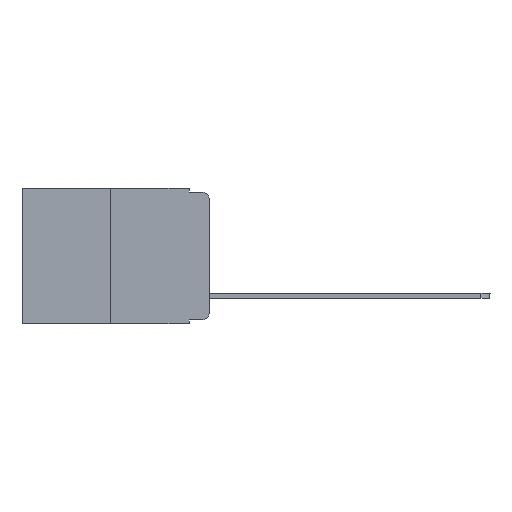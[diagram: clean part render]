
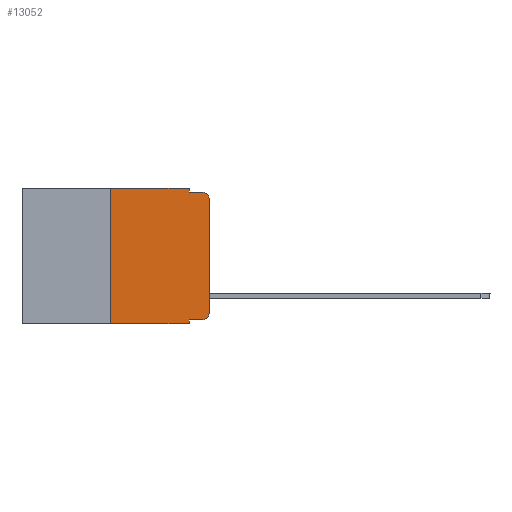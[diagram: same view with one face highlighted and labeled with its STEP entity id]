
A CAD part, left-side view. The second image highlights one B-rep face of the part: STEP entity #13052.
In plain terms, the highlighted planar face has unit normal (-1, 0, 0).
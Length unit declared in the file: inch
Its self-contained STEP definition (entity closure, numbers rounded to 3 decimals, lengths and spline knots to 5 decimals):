
#241 = DIRECTION ( 'NONE',  ( 0., 0., -1. ) ) ;
#373 = AXIS2_PLACEMENT_3D ( 'NONE', #2041, #6802, #15355 ) ;
#389 = VERTEX_POINT ( 'NONE', #5889 ) ;
#414 = EDGE_CURVE ( 'NONE', #12207, #12859, #4036, .T. ) ;
#885 = EDGE_CURVE ( 'NONE', #7667, #11808, #3461, .T. ) ;
#912 = PLANE ( 'NONE',  #373 ) ;
#1084 = DIRECTION ( 'NONE',  ( 0., 0., -1. ) ) ;
#1379 = DIRECTION ( 'NONE',  ( 0., -1., 0. ) ) ;
#1513 = CIRCLE ( 'NONE', #11182, 0.02 ) ;
#1989 = LINE ( 'NONE', #3856, #6149 ) ;
#2041 = CARTESIAN_POINT ( 'NONE',  ( 0., 0.473, 0. ) ) ;
#2101 = VERTEX_POINT ( 'NONE', #2649 ) ;
#2349 = CARTESIAN_POINT ( 'NONE',  ( 0., 0.473, 0. ) ) ;
#2479 = LINE ( 'NONE', #2349, #9505 ) ;
#2649 = CARTESIAN_POINT ( 'NONE',  ( 0., 0.02, -0.01 ) ) ;
#2656 = DIRECTION ( 'NONE',  ( 0., 0., 1. ) ) ;
#2687 = ORIENTED_EDGE ( 'NONE', *, *, #15153, .F. ) ;
#2711 = CARTESIAN_POINT ( 'NONE',  ( 0., 0.051, -0.333 ) ) ;
#3238 = CARTESIAN_POINT ( 'NONE',  ( 0., 0., -0.313 ) ) ;
#3398 = ORIENTED_EDGE ( 'NONE', *, *, #10942, .F. ) ;
#3461 = LINE ( 'NONE', #14426, #13952 ) ;
#3541 = VERTEX_POINT ( 'NONE', #10779 ) ;
#3684 = CARTESIAN_POINT ( 'NONE',  ( 0., 0.051, -0.343 ) ) ;
#3731 = EDGE_CURVE ( 'NONE', #13815, #2101, #1989, .T. ) ;
#3856 = CARTESIAN_POINT ( 'NONE',  ( 0., 0.051, -0.01 ) ) ;
#3975 = CARTESIAN_POINT ( 'NONE',  ( 0., 0.051, 0. ) ) ;
#4036 = LINE ( 'NONE', #10794, #9771 ) ;
#4743 = DIRECTION ( 'NONE',  ( -1., 0., 0. ) ) ;
#5081 = DIRECTION ( 'NONE',  ( 0., -1., 0. ) ) ;
#5144 = CARTESIAN_POINT ( 'NONE',  ( 0., 0.25, 0. ) ) ;
#5192 = ORIENTED_EDGE ( 'NONE', *, *, #9094, .F. ) ;
#5244 = VECTOR ( 'NONE', #2656, 39.37008 ) ;
#5296 = CARTESIAN_POINT ( 'NONE',  ( 0., 0.25, 0. ) ) ;
#5562 = LINE ( 'NONE', #3975, #13790 ) ;
#5621 = ORIENTED_EDGE ( 'NONE', *, *, #6258, .F. ) ;
#5871 = DIRECTION ( 'NONE',  ( 0., 0., -1. ) ) ;
#5889 = CARTESIAN_POINT ( 'NONE',  ( 0., 0.051, 0. ) ) ;
#5931 = DIRECTION ( 'NONE',  ( 0., 0., 1. ) ) ;
#6050 = DIRECTION ( 'NONE',  ( 0., -1., 0. ) ) ;
#6149 = VECTOR ( 'NONE', #5081, 39.37008 ) ;
#6258 = EDGE_CURVE ( 'NONE', #10572, #389, #2479, .T. ) ;
#6802 = DIRECTION ( 'NONE',  ( 1., 0., 0. ) ) ;
#6952 = EDGE_CURVE ( 'NONE', #11808, #2101, #8208, .T. ) ;
#7054 = ORIENTED_EDGE ( 'NONE', *, *, #11529, .T. ) ;
#7199 = VECTOR ( 'NONE', #1379, 39.37008 ) ;
#7667 = VERTEX_POINT ( 'NONE', #3238 ) ;
#7841 = ORIENTED_EDGE ( 'NONE', *, *, #3731, .F. ) ;
#8208 = CIRCLE ( 'NONE', #9423, 0.02 ) ;
#8435 = DIRECTION ( 'NONE',  ( 0., 0., -1. ) ) ;
#8578 = ORIENTED_EDGE ( 'NONE', *, *, #6952, .T. ) ;
#8870 = LINE ( 'NONE', #5144, #5244 ) ;
#9094 = EDGE_CURVE ( 'NONE', #389, #13815, #5562, .T. ) ;
#9423 = AXIS2_PLACEMENT_3D ( 'NONE', #10717, #13188, #5871 ) ;
#9505 = VECTOR ( 'NONE', #10631, 39.37008 ) ;
#9705 = LINE ( 'NONE', #14476, #15844 ) ;
#9771 = VECTOR ( 'NONE', #6050, 39.37008 ) ;
#10019 = CARTESIAN_POINT ( 'NONE',  ( 0., 0.473, -0.343 ) ) ;
#10572 = VERTEX_POINT ( 'NONE', #5296 ) ;
#10631 = DIRECTION ( 'NONE',  ( 0., -1., 0. ) ) ;
#10717 = CARTESIAN_POINT ( 'NONE',  ( 0., 0.02, -0.03 ) ) ;
#10779 = CARTESIAN_POINT ( 'NONE',  ( 0., 0.25, -0.343 ) ) ;
#10794 = CARTESIAN_POINT ( 'NONE',  ( 0., 0.051, -0.333 ) ) ;
#10815 = CARTESIAN_POINT ( 'NONE',  ( 0., 0.02, -0.313 ) ) ;
#10942 = EDGE_CURVE ( 'NONE', #12207, #11616, #9705, .T. ) ;
#11182 = AXIS2_PLACEMENT_3D ( 'NONE', #10815, #4743, #1084 ) ;
#11529 = EDGE_CURVE ( 'NONE', #12859, #7667, #1513, .T. ) ;
#11616 = VERTEX_POINT ( 'NONE', #3684 ) ;
#11798 = ORIENTED_EDGE ( 'NONE', *, *, #414, .T. ) ;
#11808 = VERTEX_POINT ( 'NONE', #13762 ) ;
#12207 = VERTEX_POINT ( 'NONE', #2711 ) ;
#12859 = VERTEX_POINT ( 'NONE', #13763 ) ;
#13052 = ADVANCED_FACE ( 'NONE', ( #13847 ), #912, .F. ) ;
#13188 = DIRECTION ( 'NONE',  ( -1., 0., 0. ) ) ;
#13210 = EDGE_LOOP ( 'NONE', ( #13373, #8578, #7841, #5192, #5621, #2687, #15255, #3398, #11798, #7054 ) ) ;
#13365 = CARTESIAN_POINT ( 'NONE',  ( 0., 0.051, -0.01 ) ) ;
#13373 = ORIENTED_EDGE ( 'NONE', *, *, #885, .T. ) ;
#13762 = CARTESIAN_POINT ( 'NONE',  ( 0., 0., -0.03 ) ) ;
#13763 = CARTESIAN_POINT ( 'NONE',  ( 0., 0.02, -0.333 ) ) ;
#13790 = VECTOR ( 'NONE', #241, 39.37008 ) ;
#13815 = VERTEX_POINT ( 'NONE', #13365 ) ;
#13847 = FACE_OUTER_BOUND ( 'NONE', #13210, .T. ) ;
#13952 = VECTOR ( 'NONE', #5931, 39.37008 ) ;
#14000 = EDGE_CURVE ( 'NONE', #3541, #11616, #14460, .T. ) ;
#14426 = CARTESIAN_POINT ( 'NONE',  ( 0., 0., 0. ) ) ;
#14460 = LINE ( 'NONE', #10019, #7199 ) ;
#14476 = CARTESIAN_POINT ( 'NONE',  ( 0., 0.051, 0. ) ) ;
#15153 = EDGE_CURVE ( 'NONE', #3541, #10572, #8870, .T. ) ;
#15255 = ORIENTED_EDGE ( 'NONE', *, *, #14000, .T. ) ;
#15355 = DIRECTION ( 'NONE',  ( 0., 0., -1. ) ) ;
#15844 = VECTOR ( 'NONE', #8435, 39.37008 ) ;
